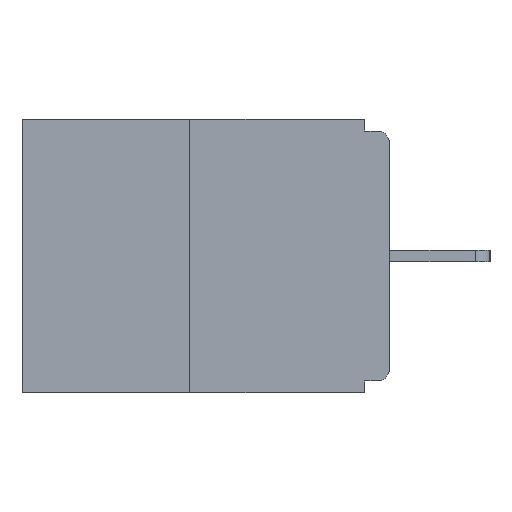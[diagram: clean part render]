
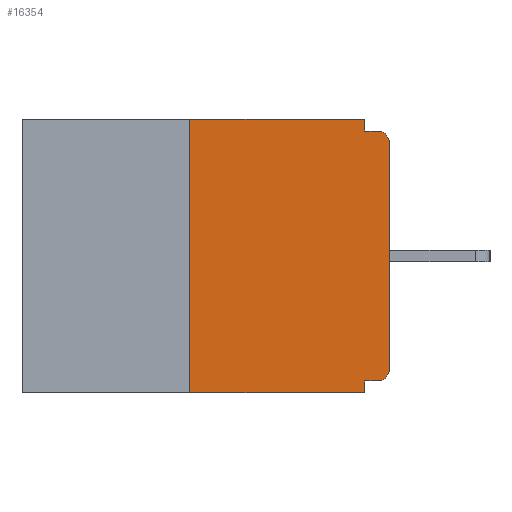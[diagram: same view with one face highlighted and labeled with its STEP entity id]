
A CAD part, left-side view. The second image highlights one B-rep face of the part: STEP entity #16354.
In plain terms, the highlighted planar face has unit normal (-1, 0, 0).
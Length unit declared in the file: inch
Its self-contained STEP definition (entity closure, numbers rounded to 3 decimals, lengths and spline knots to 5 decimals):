
#194 = FACE_OUTER_BOUND ( 'NONE', #1913, .T. ) ;
#402 = DIRECTION ( 'NONE',  ( 0., -1., 0. ) ) ;
#846 = EDGE_CURVE ( 'NONE', #14664, #16108, #16980, .T. ) ;
#866 = EDGE_CURVE ( 'NONE', #19988, #9576, #20097, .T. ) ;
#1165 = VERTEX_POINT ( 'NONE', #6442 ) ;
#1184 = DIRECTION ( 'NONE',  ( 0., 0., -1. ) ) ;
#1572 = EDGE_CURVE ( 'NONE', #5525, #14664, #8856, .T. ) ;
#1913 = EDGE_LOOP ( 'NONE', ( #19234, #12897, #5170, #5618, #13598, #10048, #2182, #9368, #7354, #11366 ) ) ;
#1955 = VECTOR ( 'NONE', #5914, 39.37008 ) ;
#2163 = CIRCLE ( 'NONE', #17098, 0.015 ) ;
#2182 = ORIENTED_EDGE ( 'NONE', *, *, #1572, .T. ) ;
#2378 = CARTESIAN_POINT ( 'NONE',  ( 0., 0.015, -0.015 ) ) ;
#2400 = DIRECTION ( 'NONE',  ( -1., 0., 0. ) ) ;
#2490 = CARTESIAN_POINT ( 'NONE',  ( 0., 0.031, -0.015 ) ) ;
#2816 = CARTESIAN_POINT ( 'NONE',  ( 0., 0.031, -0.343 ) ) ;
#2950 = CARTESIAN_POINT ( 'NONE',  ( 0., 0., -0.015 ) ) ;
#3485 = VERTEX_POINT ( 'NONE', #20015 ) ;
#3711 = LINE ( 'NONE', #13357, #5006 ) ;
#3947 = LINE ( 'NONE', #4259, #14401 ) ;
#3964 = EDGE_CURVE ( 'NONE', #1165, #5525, #2163, .T. ) ;
#4098 = CARTESIAN_POINT ( 'NONE',  ( 0., 0., -0.313 ) ) ;
#4099 = AXIS2_PLACEMENT_3D ( 'NONE', #19452, #6366, #11151 ) ;
#4259 = CARTESIAN_POINT ( 'NONE',  ( 0., 0.46, -0.343 ) ) ;
#4880 = DIRECTION ( 'NONE',  ( 0., 0., -1. ) ) ;
#5006 = VECTOR ( 'NONE', #4880, 39.37008 ) ;
#5047 = EDGE_CURVE ( 'NONE', #3485, #10572, #3947, .T. ) ;
#5170 = ORIENTED_EDGE ( 'NONE', *, *, #5047, .T. ) ;
#5525 = VERTEX_POINT ( 'NONE', #4098 ) ;
#5618 = ORIENTED_EDGE ( 'NONE', *, *, #13446, .F. ) ;
#5914 = DIRECTION ( 'NONE',  ( 0., -1., 0. ) ) ;
#6366 = DIRECTION ( 'NONE',  ( -1., 0., 0. ) ) ;
#6442 = CARTESIAN_POINT ( 'NONE',  ( 0., 0.015, -0.328 ) ) ;
#6514 = LINE ( 'NONE', #17701, #8354 ) ;
#6853 = VERTEX_POINT ( 'NONE', #2490 ) ;
#7354 = ORIENTED_EDGE ( 'NONE', *, *, #9575, .F. ) ;
#7442 = EDGE_CURVE ( 'NONE', #3485, #19988, #16169, .T. ) ;
#7526 = DIRECTION ( 'NONE',  ( 0., -1., 0. ) ) ;
#7655 = LINE ( 'NONE', #17263, #12347 ) ;
#8257 = PLANE ( 'NONE',  #15468 ) ;
#8354 = VECTOR ( 'NONE', #21011, 39.37008 ) ;
#8366 = DIRECTION ( 'NONE',  ( 1., 0., 0. ) ) ;
#8856 = LINE ( 'NONE', #20265, #21006 ) ;
#9287 = EDGE_CURVE ( 'NONE', #9576, #6853, #3711, .T. ) ;
#9368 = ORIENTED_EDGE ( 'NONE', *, *, #846, .T. ) ;
#9575 = EDGE_CURVE ( 'NONE', #6853, #16108, #13986, .T. ) ;
#9576 = VERTEX_POINT ( 'NONE', #12377 ) ;
#10048 = ORIENTED_EDGE ( 'NONE', *, *, #3964, .T. ) ;
#10074 = CARTESIAN_POINT ( 'NONE',  ( 0., 0.46, 0. ) ) ;
#10572 = VERTEX_POINT ( 'NONE', #2816 ) ;
#11151 = DIRECTION ( 'NONE',  ( 0., 0., -1. ) ) ;
#11366 = ORIENTED_EDGE ( 'NONE', *, *, #9287, .F. ) ;
#11458 = CARTESIAN_POINT ( 'NONE',  ( 0., 0.25, 0. ) ) ;
#11843 = DIRECTION ( 'NONE',  ( 0., 0., -1. ) ) ;
#12042 = CARTESIAN_POINT ( 'NONE',  ( 0., 0.015, -0.313 ) ) ;
#12347 = VECTOR ( 'NONE', #1184, 39.37008 ) ;
#12377 = CARTESIAN_POINT ( 'NONE',  ( 0., 0.031, 0. ) ) ;
#12897 = ORIENTED_EDGE ( 'NONE', *, *, #7442, .F. ) ;
#13357 = CARTESIAN_POINT ( 'NONE',  ( 0., 0.031, 0. ) ) ;
#13446 = EDGE_CURVE ( 'NONE', #18486, #10572, #7655, .T. ) ;
#13598 = ORIENTED_EDGE ( 'NONE', *, *, #17893, .F. ) ;
#13603 = VECTOR ( 'NONE', #402, 39.37008 ) ;
#13643 = DIRECTION ( 'NONE',  ( 0., 0., 1. ) ) ;
#13888 = CARTESIAN_POINT ( 'NONE',  ( 0., 0.031, -0.328 ) ) ;
#13986 = LINE ( 'NONE', #2950, #1955 ) ;
#14401 = VECTOR ( 'NONE', #7526, 39.37008 ) ;
#14664 = VERTEX_POINT ( 'NONE', #17772 ) ;
#15468 = AXIS2_PLACEMENT_3D ( 'NONE', #10074, #8366, #19884 ) ;
#15857 = VECTOR ( 'NONE', #20860, 39.37008 ) ;
#16108 = VERTEX_POINT ( 'NONE', #2378 ) ;
#16169 = LINE ( 'NONE', #19062, #15857 ) ;
#16354 = ADVANCED_FACE ( 'NONE', ( #194 ), #8257, .F. ) ;
#16980 = CIRCLE ( 'NONE', #4099, 0.015 ) ;
#17098 = AXIS2_PLACEMENT_3D ( 'NONE', #12042, #2400, #11843 ) ;
#17263 = CARTESIAN_POINT ( 'NONE',  ( 0., 0.031, -0.343 ) ) ;
#17701 = CARTESIAN_POINT ( 'NONE',  ( 0., 0., -0.328 ) ) ;
#17772 = CARTESIAN_POINT ( 'NONE',  ( 0., 0., -0.03 ) ) ;
#17893 = EDGE_CURVE ( 'NONE', #1165, #18486, #6514, .T. ) ;
#18166 = CARTESIAN_POINT ( 'NONE',  ( 0., 0.46, 0. ) ) ;
#18486 = VERTEX_POINT ( 'NONE', #13888 ) ;
#19062 = CARTESIAN_POINT ( 'NONE',  ( 0., 0.25, 0. ) ) ;
#19234 = ORIENTED_EDGE ( 'NONE', *, *, #866, .F. ) ;
#19452 = CARTESIAN_POINT ( 'NONE',  ( 0., 0.015, -0.03 ) ) ;
#19884 = DIRECTION ( 'NONE',  ( 0., 0., -1. ) ) ;
#19988 = VERTEX_POINT ( 'NONE', #11458 ) ;
#20015 = CARTESIAN_POINT ( 'NONE',  ( 0., 0.25, -0.343 ) ) ;
#20097 = LINE ( 'NONE', #18166, #13603 ) ;
#20265 = CARTESIAN_POINT ( 'NONE',  ( 0., 0., 0. ) ) ;
#20860 = DIRECTION ( 'NONE',  ( 0., 0., 1. ) ) ;
#21006 = VECTOR ( 'NONE', #13643, 39.37008 ) ;
#21011 = DIRECTION ( 'NONE',  ( 0., 1., 0. ) ) ;
